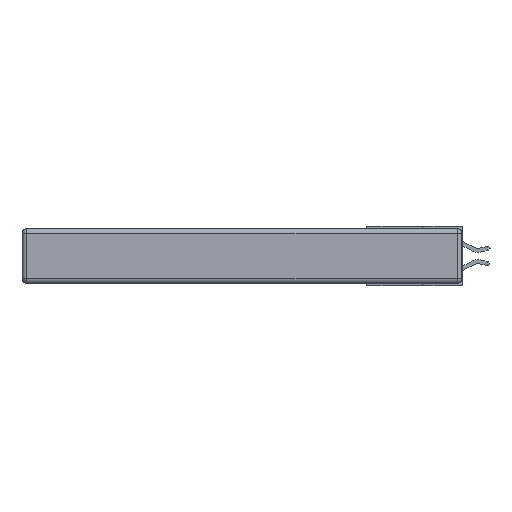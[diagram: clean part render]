
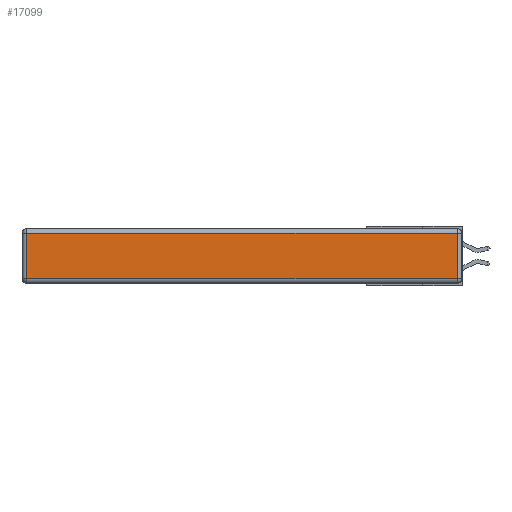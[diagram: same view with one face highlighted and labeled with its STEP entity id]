
A CAD part, left-side view. The second image highlights one B-rep face of the part: STEP entity #17099.
In plain terms, the highlighted planar face has unit normal (-1, 0, 0).
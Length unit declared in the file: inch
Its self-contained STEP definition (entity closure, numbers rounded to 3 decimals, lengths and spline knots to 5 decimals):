
#1171 = LINE ( 'NONE', #2006, #3460 ) ;
#2006 = CARTESIAN_POINT ( 'NONE',  ( 0., 0.03, -0.343 ) ) ;
#2641 = ORIENTED_EDGE ( 'NONE', *, *, #4650, .T. ) ;
#2699 = EDGE_CURVE ( 'NONE', #3901, #8955, #11625, .T. ) ;
#3460 = VECTOR ( 'NONE', #5298, 39.37008 ) ;
#3529 = DIRECTION ( 'NONE',  ( 0., 0., -1. ) ) ;
#3680 = ORIENTED_EDGE ( 'NONE', *, *, #18257, .T. ) ;
#3901 = VERTEX_POINT ( 'NONE', #14513 ) ;
#3944 = CARTESIAN_POINT ( 'NONE',  ( 0., 0., -0.343 ) ) ;
#4650 = EDGE_CURVE ( 'NONE', #10649, #3901, #9690, .T. ) ;
#5298 = DIRECTION ( 'NONE',  ( 0., 0., 1. ) ) ;
#5615 = DIRECTION ( 'NONE',  ( 0., 0., 1. ) ) ;
#5699 = ORIENTED_EDGE ( 'NONE', *, *, #2699, .T. ) ;
#6047 = VECTOR ( 'NONE', #7114, 39.37008 ) ;
#6357 = EDGE_LOOP ( 'NONE', ( #5699, #13708, #3680, #2641 ) ) ;
#7114 = DIRECTION ( 'NONE',  ( 0., 1., 0. ) ) ;
#8418 = FACE_OUTER_BOUND ( 'NONE', #6357, .T. ) ;
#8955 = VERTEX_POINT ( 'NONE', #16366 ) ;
#9230 = CARTESIAN_POINT ( 'NONE',  ( 0., 0., -0.313 ) ) ;
#9690 = LINE ( 'NONE', #12880, #17966 ) ;
#10055 = VECTOR ( 'NONE', #12303, 39.37008 ) ;
#10649 = VERTEX_POINT ( 'NONE', #21095 ) ;
#11625 = LINE ( 'NONE', #9230, #10055 ) ;
#12303 = DIRECTION ( 'NONE',  ( 0., -1., 0. ) ) ;
#12593 = CARTESIAN_POINT ( 'NONE',  ( 0., 0.03, -0.03 ) ) ;
#12880 = CARTESIAN_POINT ( 'NONE',  ( 0., 2.72, -0.343 ) ) ;
#13708 = ORIENTED_EDGE ( 'NONE', *, *, #17696, .T. ) ;
#13815 = PLANE ( 'NONE',  #16822 ) ;
#14513 = CARTESIAN_POINT ( 'NONE',  ( 0., 2.72, -0.313 ) ) ;
#15547 = DIRECTION ( 'NONE',  ( -1., 0., 0. ) ) ;
#16366 = CARTESIAN_POINT ( 'NONE',  ( 0., 0.03, -0.313 ) ) ;
#16822 = AXIS2_PLACEMENT_3D ( 'NONE', #3944, #15547, #5615 ) ;
#16998 = CARTESIAN_POINT ( 'NONE',  ( 0., 2.75, -0.03 ) ) ;
#17099 = ADVANCED_FACE ( 'NONE', ( #8418 ), #13815, .T. ) ;
#17696 = EDGE_CURVE ( 'NONE', #8955, #19543, #1171, .T. ) ;
#17966 = VECTOR ( 'NONE', #3529, 39.37008 ) ;
#18257 = EDGE_CURVE ( 'NONE', #19543, #10649, #18714, .T. ) ;
#18714 = LINE ( 'NONE', #16998, #6047 ) ;
#19543 = VERTEX_POINT ( 'NONE', #12593 ) ;
#21095 = CARTESIAN_POINT ( 'NONE',  ( 0., 2.72, -0.03 ) ) ;
